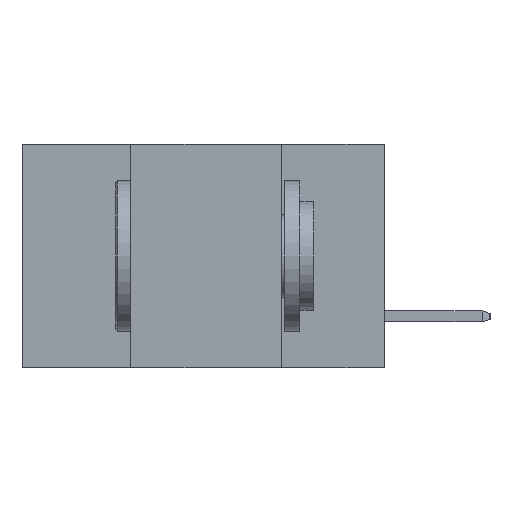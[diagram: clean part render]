
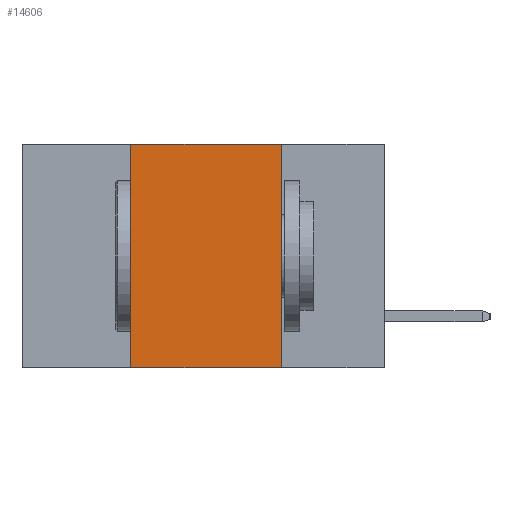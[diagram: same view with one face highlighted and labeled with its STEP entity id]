
A CAD part, left-side view. The second image highlights one B-rep face of the part: STEP entity #14606.
In plain terms, the highlighted planar face has unit normal (-1, 0, 0).
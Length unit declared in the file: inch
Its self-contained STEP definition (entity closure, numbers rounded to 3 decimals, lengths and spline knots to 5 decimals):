
#213 = LINE ( 'NONE', #3986, #19000 ) ;
#526 = CARTESIAN_POINT ( 'NONE',  ( 0., 0.17, 0. ) ) ;
#782 = DIRECTION ( 'NONE',  ( 0., -1., 0. ) ) ;
#1017 = CARTESIAN_POINT ( 'NONE',  ( 0., 0.42, -0.37 ) ) ;
#1259 = ORIENTED_EDGE ( 'NONE', *, *, #20857, .F. ) ;
#1508 = CARTESIAN_POINT ( 'NONE',  ( 0., 0.17, -0.37 ) ) ;
#2313 = CARTESIAN_POINT ( 'NONE',  ( 0., 0.42, 0. ) ) ;
#2584 = VECTOR ( 'NONE', #14149, 39.37008 ) ;
#3738 = EDGE_CURVE ( 'NONE', #13055, #22624, #9561, .T. ) ;
#3986 = CARTESIAN_POINT ( 'NONE',  ( 0., 0.42, 0. ) ) ;
#4142 = AXIS2_PLACEMENT_3D ( 'NONE', #23235, #17916, #7133 ) ;
#4351 = CARTESIAN_POINT ( 'NONE',  ( 0., 0.17, 0. ) ) ;
#4675 = DIRECTION ( 'NONE',  ( 0., 0., -1. ) ) ;
#5259 = PLANE ( 'NONE',  #4142 ) ;
#5484 = EDGE_LOOP ( 'NONE', ( #5888, #16082, #1259, #21738 ) ) ;
#5888 = ORIENTED_EDGE ( 'NONE', *, *, #3738, .F. ) ;
#6961 = CARTESIAN_POINT ( 'NONE',  ( 0., 0.6, -0.37 ) ) ;
#7133 = DIRECTION ( 'NONE',  ( 0., 0., -1. ) ) ;
#9506 = DIRECTION ( 'NONE',  ( 0., 0., 1. ) ) ;
#9561 = LINE ( 'NONE', #526, #18007 ) ;
#9697 = EDGE_CURVE ( 'NONE', #18353, #13055, #13299, .T. ) ;
#9768 = VERTEX_POINT ( 'NONE', #1017 ) ;
#11159 = LINE ( 'NONE', #6961, #2584 ) ;
#12734 = VECTOR ( 'NONE', #782, 39.37008 ) ;
#13055 = VERTEX_POINT ( 'NONE', #4351 ) ;
#13299 = LINE ( 'NONE', #17128, #12734 ) ;
#14149 = DIRECTION ( 'NONE',  ( 0., -1., 0. ) ) ;
#14606 = ADVANCED_FACE ( 'NONE', ( #15851 ), #5259, .F. ) ;
#15851 = FACE_OUTER_BOUND ( 'NONE', #5484, .T. ) ;
#16082 = ORIENTED_EDGE ( 'NONE', *, *, #9697, .F. ) ;
#17128 = CARTESIAN_POINT ( 'NONE',  ( 0., 0.6, 0. ) ) ;
#17916 = DIRECTION ( 'NONE',  ( 1., 0., 0. ) ) ;
#18007 = VECTOR ( 'NONE', #4675, 39.37008 ) ;
#18353 = VERTEX_POINT ( 'NONE', #2313 ) ;
#19000 = VECTOR ( 'NONE', #9506, 39.37008 ) ;
#19970 = EDGE_CURVE ( 'NONE', #9768, #22624, #11159, .T. ) ;
#20857 = EDGE_CURVE ( 'NONE', #9768, #18353, #213, .T. ) ;
#21738 = ORIENTED_EDGE ( 'NONE', *, *, #19970, .T. ) ;
#22624 = VERTEX_POINT ( 'NONE', #1508 ) ;
#23235 = CARTESIAN_POINT ( 'NONE',  ( 0., 0.6, 0. ) ) ;
